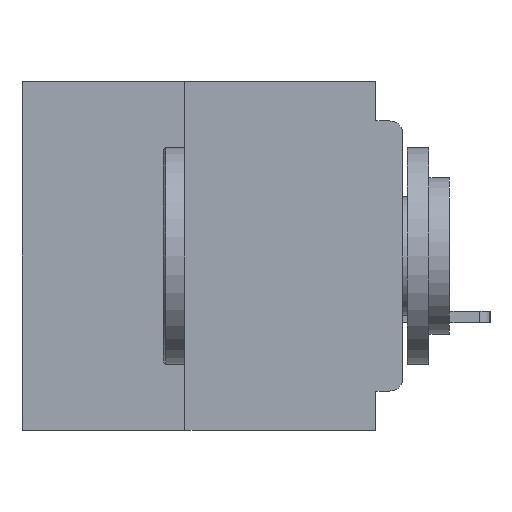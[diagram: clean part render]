
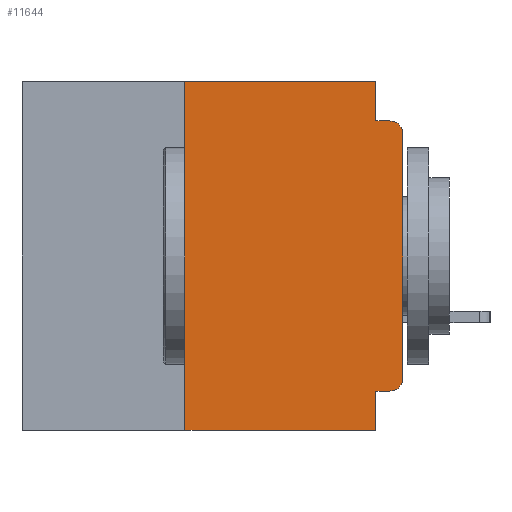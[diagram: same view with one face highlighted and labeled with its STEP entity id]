
A CAD part, left-side view. The second image highlights one B-rep face of the part: STEP entity #11644.
In plain terms, the highlighted planar face has unit normal (-1, 0, 0).
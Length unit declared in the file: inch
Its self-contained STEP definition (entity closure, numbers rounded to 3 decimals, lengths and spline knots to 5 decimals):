
#1144 = EDGE_CURVE ( 'NONE', #5641, #22174, #31620, .T. ) ;
#1645 = EDGE_CURVE ( 'NONE', #48306, #22614, #36967, .T. ) ;
#1706 = VECTOR ( 'NONE', #7542, 39.37008 ) ;
#1854 = VERTEX_POINT ( 'NONE', #40935 ) ;
#2069 = EDGE_CURVE ( 'NONE', #14868, #48306, #25512, .T. ) ;
#3618 = CARTESIAN_POINT ( 'NONE',  ( 0., 0.015, -0.355 ) ) ;
#3703 = CARTESIAN_POINT ( 'NONE',  ( 0., 0., -0.045 ) ) ;
#3888 = ORIENTED_EDGE ( 'NONE', *, *, #28188, .T. ) ;
#3999 = CARTESIAN_POINT ( 'NONE',  ( 0., 0.031, -0.045 ) ) ;
#5278 = ORIENTED_EDGE ( 'NONE', *, *, #1645, .F. ) ;
#5486 = VERTEX_POINT ( 'NONE', #21827 ) ;
#5641 = VERTEX_POINT ( 'NONE', #49295 ) ;
#6004 = VECTOR ( 'NONE', #36947, 39.37008 ) ;
#6470 = AXIS2_PLACEMENT_3D ( 'NONE', #24268, #39700, #16742 ) ;
#6933 = EDGE_CURVE ( 'NONE', #22614, #22174, #23270, .T. ) ;
#7542 = DIRECTION ( 'NONE',  ( 0., -1., 0. ) ) ;
#7734 = LINE ( 'NONE', #11374, #37112 ) ;
#8048 = ORIENTED_EDGE ( 'NONE', *, *, #42542, .T. ) ;
#9746 = CARTESIAN_POINT ( 'NONE',  ( 0., 0.437, -0.4 ) ) ;
#9901 = CARTESIAN_POINT ( 'NONE',  ( 0., 0.25, -0.4 ) ) ;
#10547 = ORIENTED_EDGE ( 'NONE', *, *, #2069, .F. ) ;
#11115 = AXIS2_PLACEMENT_3D ( 'NONE', #22796, #49435, #26631 ) ;
#11374 = CARTESIAN_POINT ( 'NONE',  ( 0., 0.25, -0.4 ) ) ;
#11644 = ADVANCED_FACE ( 'NONE', ( #34907 ), #35849, .F. ) ;
#13020 = EDGE_CURVE ( 'NONE', #1854, #5486, #38945, .T. ) ;
#13596 = CARTESIAN_POINT ( 'NONE',  ( 0., 0.031, -0.4 ) ) ;
#14233 = VECTOR ( 'NONE', #26342, 39.37008 ) ;
#14798 = CIRCLE ( 'NONE', #11115, 0.015 ) ;
#14868 = VERTEX_POINT ( 'NONE', #47121 ) ;
#16149 = ORIENTED_EDGE ( 'NONE', *, *, #29371, .F. ) ;
#16532 = VECTOR ( 'NONE', #32947, 39.37008 ) ;
#16575 = VECTOR ( 'NONE', #46896, 39.37008 ) ;
#16742 = DIRECTION ( 'NONE',  ( 0., 0., -1. ) ) ;
#17342 = LINE ( 'NONE', #9746, #35354 ) ;
#17466 = DIRECTION ( 'NONE',  ( 0., -1., 0. ) ) ;
#19204 = VERTEX_POINT ( 'NONE', #9901 ) ;
#19707 = CARTESIAN_POINT ( 'NONE',  ( 0., 0., -0.34 ) ) ;
#19709 = ORIENTED_EDGE ( 'NONE', *, *, #1144, .T. ) ;
#21827 = CARTESIAN_POINT ( 'NONE',  ( 0., 0.031, -0.4 ) ) ;
#22174 = VERTEX_POINT ( 'NONE', #28302 ) ;
#22614 = VERTEX_POINT ( 'NONE', #3999 ) ;
#22796 = CARTESIAN_POINT ( 'NONE',  ( 0., 0.015, -0.34 ) ) ;
#22988 = EDGE_CURVE ( 'NONE', #27948, #5641, #36562, .T. ) ;
#23270 = LINE ( 'NONE', #3703, #1706 ) ;
#24268 = CARTESIAN_POINT ( 'NONE',  ( 0., 0.437, 0. ) ) ;
#25512 = LINE ( 'NONE', #33009, #16532 ) ;
#26342 = DIRECTION ( 'NONE',  ( 0., 1., 0. ) ) ;
#26631 = DIRECTION ( 'NONE',  ( 0., 0., -1. ) ) ;
#27948 = VERTEX_POINT ( 'NONE', #19707 ) ;
#28132 = ORIENTED_EDGE ( 'NONE', *, *, #22988, .T. ) ;
#28188 = EDGE_CURVE ( 'NONE', #19204, #5486, #17342, .T. ) ;
#28302 = CARTESIAN_POINT ( 'NONE',  ( 0., 0.015, -0.045 ) ) ;
#29371 = EDGE_CURVE ( 'NONE', #33454, #1854, #33434, .T. ) ;
#30765 = CARTESIAN_POINT ( 'NONE',  ( 0., 0.031, 0. ) ) ;
#31620 = CIRCLE ( 'NONE', #38049, 0.015 ) ;
#32695 = DIRECTION ( 'NONE',  ( 0., 0., -1. ) ) ;
#32947 = DIRECTION ( 'NONE',  ( 0., -1., 0. ) ) ;
#33009 = CARTESIAN_POINT ( 'NONE',  ( 0., 0.437, 0. ) ) ;
#33089 = CARTESIAN_POINT ( 'NONE',  ( 0., 0., 0. ) ) ;
#33280 = DIRECTION ( 'NONE',  ( 0., 0., -1. ) ) ;
#33352 = DIRECTION ( 'NONE',  ( -1., 0., 0. ) ) ;
#33434 = LINE ( 'NONE', #45410, #14233 ) ;
#33454 = VERTEX_POINT ( 'NONE', #3618 ) ;
#33629 = CARTESIAN_POINT ( 'NONE',  ( 0., 0.015, -0.06 ) ) ;
#34358 = DIRECTION ( 'NONE',  ( 0., 0., 1. ) ) ;
#34907 = FACE_OUTER_BOUND ( 'NONE', #44694, .T. ) ;
#35354 = VECTOR ( 'NONE', #17466, 39.37008 ) ;
#35730 = ORIENTED_EDGE ( 'NONE', *, *, #6933, .F. ) ;
#35849 = PLANE ( 'NONE',  #6470 ) ;
#36278 = EDGE_CURVE ( 'NONE', #19204, #14868, #7734, .T. ) ;
#36562 = LINE ( 'NONE', #33089, #6004 ) ;
#36947 = DIRECTION ( 'NONE',  ( 0., 0., 1. ) ) ;
#36967 = LINE ( 'NONE', #46953, #16575 ) ;
#37112 = VECTOR ( 'NONE', #34358, 39.37008 ) ;
#37729 = VECTOR ( 'NONE', #32695, 39.37008 ) ;
#38049 = AXIS2_PLACEMENT_3D ( 'NONE', #33629, #33352, #33280 ) ;
#38945 = LINE ( 'NONE', #13596, #37729 ) ;
#39700 = DIRECTION ( 'NONE',  ( 1., 0., 0. ) ) ;
#40935 = CARTESIAN_POINT ( 'NONE',  ( 0., 0.031, -0.355 ) ) ;
#42542 = EDGE_CURVE ( 'NONE', #33454, #27948, #14798, .T. ) ;
#42748 = ORIENTED_EDGE ( 'NONE', *, *, #36278, .F. ) ;
#44694 = EDGE_LOOP ( 'NONE', ( #28132, #19709, #35730, #5278, #10547, #42748, #3888, #44860, #16149, #8048 ) ) ;
#44860 = ORIENTED_EDGE ( 'NONE', *, *, #13020, .F. ) ;
#45410 = CARTESIAN_POINT ( 'NONE',  ( 0., 0., -0.355 ) ) ;
#46896 = DIRECTION ( 'NONE',  ( 0., 0., -1. ) ) ;
#46953 = CARTESIAN_POINT ( 'NONE',  ( 0., 0.031, 0. ) ) ;
#47121 = CARTESIAN_POINT ( 'NONE',  ( 0., 0.25, 0. ) ) ;
#48306 = VERTEX_POINT ( 'NONE', #30765 ) ;
#49295 = CARTESIAN_POINT ( 'NONE',  ( 0., 0., -0.06 ) ) ;
#49435 = DIRECTION ( 'NONE',  ( -1., 0., 0. ) ) ;
